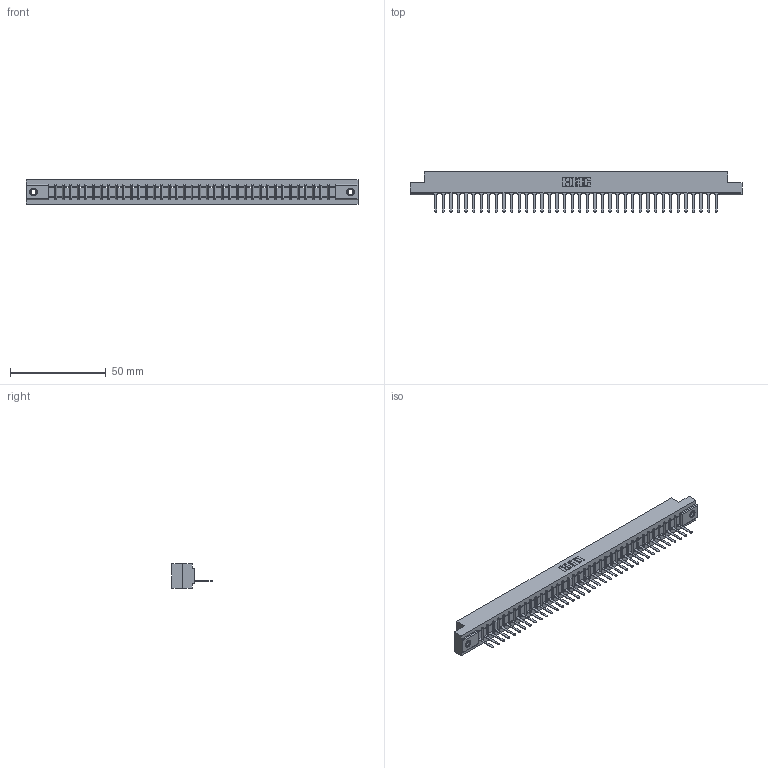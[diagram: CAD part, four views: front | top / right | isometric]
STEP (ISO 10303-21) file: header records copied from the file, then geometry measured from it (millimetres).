
FILE_DESCRIPTION (( 'STEP AP203' ), '1' );
FILE_NAME ('357-038-527-107.STEP', '2018-08-10T08:29:17', ( '' ), ( '' ), 'SwSTEP 2.0', 'SolidWorks 2016', '' );
FILE_SCHEMA (( 'CONFIG_CONTROL_DESIGN' ));
Length unit declared in the file: inch
Products named in the file (4): 307 Part_.156 Dia Mounting Holes; 307-290-001_527; 345-250-001_345-250-005-103; 357-038-527-107
Assembly tree (41 placements, depth 2):
  357-038-527-107
    307 Part_.156 Dia Mounting Holes
    307-290-001_527  x38
    345-250-001_345-250-005-103  x2
Bounding box: 173.58 x 21.11 x 12.7 mm (x, y, z)
Volume: 18008.3 mm3; surface area: 19182.6 mm2
Topology: 41 solids, 41 shells, 2345 faces, 6615 edges, 4246 vertices
Faces by surface type: plane 1508, cylinder 743, sphere 78, cone 12, torus 4
Entity records: 34223 total; most frequent: CARTESIAN_POINT 5743, ORIENTED_EDGE 5722, DIRECTION 5597, EDGE_CURVE 2861, LINE 2193, VECTOR 2193, VERTEX_POINT 1848, AXIS2_PLACEMENT_3D 1702
